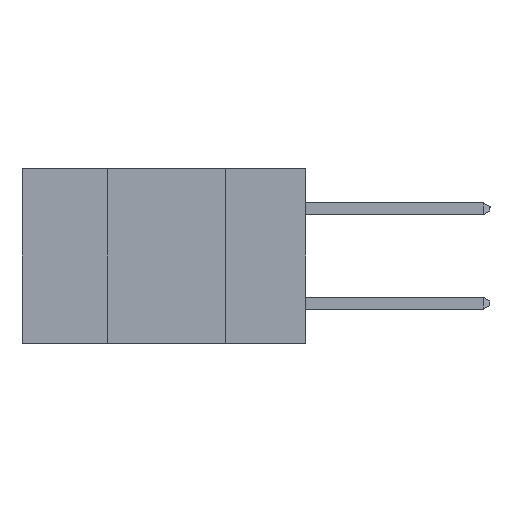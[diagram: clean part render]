
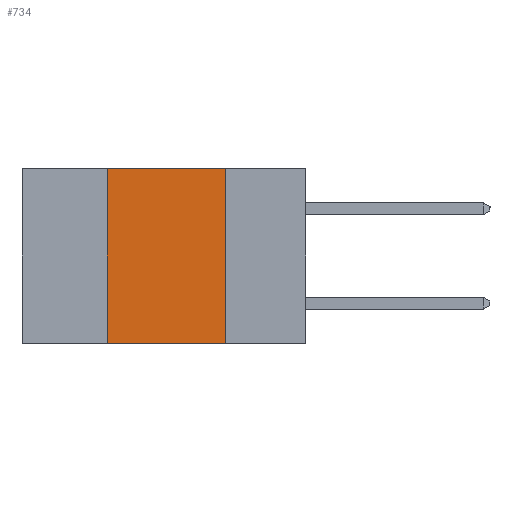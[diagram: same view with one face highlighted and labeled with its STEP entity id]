
A CAD part, left-side view. The second image highlights one B-rep face of the part: STEP entity #734.
In plain terms, the highlighted planar face has unit normal (-1, 0, 0).
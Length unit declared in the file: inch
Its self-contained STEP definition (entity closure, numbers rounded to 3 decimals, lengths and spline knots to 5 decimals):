
#98 = LINE ( 'NONE', #13958, #5782 ) ;
#457 = CARTESIAN_POINT ( 'NONE',  ( 0., 0.17, -0.37 ) ) ;
#734 = ADVANCED_FACE ( 'NONE', ( #12671 ), #11291, .F. ) ;
#957 = CARTESIAN_POINT ( 'NONE',  ( 0., 0.42, -0.37 ) ) ;
#2862 = VERTEX_POINT ( 'NONE', #3707 ) ;
#2904 = CARTESIAN_POINT ( 'NONE',  ( 0., 0.6, 0. ) ) ;
#2947 = VECTOR ( 'NONE', #4194, 39.37008 ) ;
#3000 = CARTESIAN_POINT ( 'NONE',  ( 0., 0.6, -0.37 ) ) ;
#3651 = DIRECTION ( 'NONE',  ( 0., 0., -1. ) ) ;
#3707 = CARTESIAN_POINT ( 'NONE',  ( 0., 0.17, 0. ) ) ;
#4172 = DIRECTION ( 'NONE',  ( 0., -1., 0. ) ) ;
#4194 = DIRECTION ( 'NONE',  ( 0., -1., 0. ) ) ;
#4207 = VERTEX_POINT ( 'NONE', #12052 ) ;
#4216 = ORIENTED_EDGE ( 'NONE', *, *, #9331, .F. ) ;
#4594 = VERTEX_POINT ( 'NONE', #457 ) ;
#5507 = DIRECTION ( 'NONE',  ( 0., 0., -1. ) ) ;
#5580 = CARTESIAN_POINT ( 'NONE',  ( 0., 0.6, 0. ) ) ;
#5782 = VECTOR ( 'NONE', #3651, 39.37008 ) ;
#6492 = AXIS2_PLACEMENT_3D ( 'NONE', #5580, #11222, #5507 ) ;
#7398 = LINE ( 'NONE', #2904, #8245 ) ;
#7576 = ORIENTED_EDGE ( 'NONE', *, *, #12413, .F. ) ;
#7696 = ORIENTED_EDGE ( 'NONE', *, *, #8730, .F. ) ;
#8015 = DIRECTION ( 'NONE',  ( 0., 0., 1. ) ) ;
#8206 = ORIENTED_EDGE ( 'NONE', *, *, #10310, .T. ) ;
#8245 = VECTOR ( 'NONE', #4172, 39.37008 ) ;
#8730 = EDGE_CURVE ( 'NONE', #14240, #4207, #12327, .T. ) ;
#8814 = CARTESIAN_POINT ( 'NONE',  ( 0., 0.42, -0.37 ) ) ;
#9331 = EDGE_CURVE ( 'NONE', #2862, #4594, #98, .T. ) ;
#9861 = VECTOR ( 'NONE', #8015, 39.37008 ) ;
#10310 = EDGE_CURVE ( 'NONE', #14240, #4594, #12089, .T. ) ;
#11222 = DIRECTION ( 'NONE',  ( 1., 0., 0. ) ) ;
#11291 = PLANE ( 'NONE',  #6492 ) ;
#12052 = CARTESIAN_POINT ( 'NONE',  ( 0., 0.42, 0. ) ) ;
#12089 = LINE ( 'NONE', #3000, #2947 ) ;
#12327 = LINE ( 'NONE', #957, #9861 ) ;
#12365 = EDGE_LOOP ( 'NONE', ( #4216, #7576, #7696, #8206 ) ) ;
#12413 = EDGE_CURVE ( 'NONE', #4207, #2862, #7398, .T. ) ;
#12671 = FACE_OUTER_BOUND ( 'NONE', #12365, .T. ) ;
#13958 = CARTESIAN_POINT ( 'NONE',  ( 0., 0.17, -0.37 ) ) ;
#14240 = VERTEX_POINT ( 'NONE', #8814 ) ;
